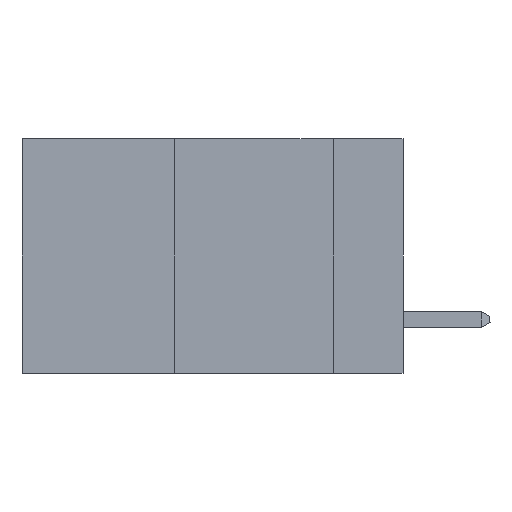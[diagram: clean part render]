
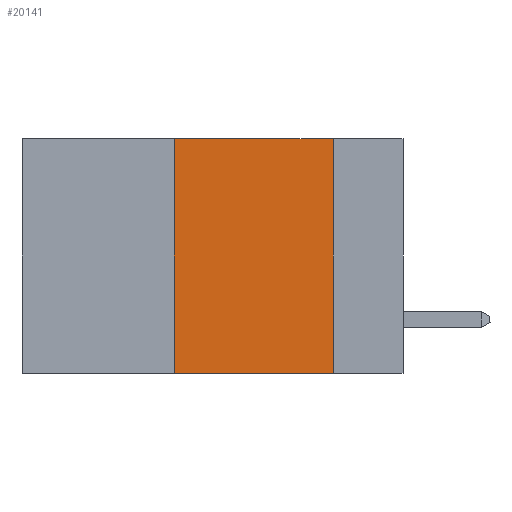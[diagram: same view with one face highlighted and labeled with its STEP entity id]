
A CAD part, left-side view. The second image highlights one B-rep face of the part: STEP entity #20141.
In plain terms, the highlighted planar face has unit normal (-1, 0, 0).
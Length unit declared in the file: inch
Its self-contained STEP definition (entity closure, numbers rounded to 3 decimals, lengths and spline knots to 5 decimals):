
#203 = VERTEX_POINT ( 'NONE', #24056 ) ;
#436 = DIRECTION ( 'NONE',  ( 0., 0., -1. ) ) ;
#682 = LINE ( 'NONE', #20265, #16203 ) ;
#1574 = ORIENTED_EDGE ( 'NONE', *, *, #17843, .F. ) ;
#2087 = CARTESIAN_POINT ( 'NONE',  ( 0., 0.6, 0. ) ) ;
#3830 = EDGE_CURVE ( 'NONE', #203, #29675, #9218, .T. ) ;
#4509 = CARTESIAN_POINT ( 'NONE',  ( 0., 0.6, -0.37 ) ) ;
#5100 = CARTESIAN_POINT ( 'NONE',  ( 0., 0.11, -0.37 ) ) ;
#5851 = CARTESIAN_POINT ( 'NONE',  ( 0., 0.36, 0. ) ) ;
#6160 = AXIS2_PLACEMENT_3D ( 'NONE', #2087, #24772, #436 ) ;
#6168 = ORIENTED_EDGE ( 'NONE', *, *, #24095, .F. ) ;
#7681 = CARTESIAN_POINT ( 'NONE',  ( 0., 0.6, 0. ) ) ;
#9218 = LINE ( 'NONE', #5851, #25414 ) ;
#9729 = DIRECTION ( 'NONE',  ( 0., -1., 0. ) ) ;
#9740 = VERTEX_POINT ( 'NONE', #19807 ) ;
#10594 = VECTOR ( 'NONE', #11298, 39.37008 ) ;
#11052 = CARTESIAN_POINT ( 'NONE',  ( 0., 0.36, 0. ) ) ;
#11298 = DIRECTION ( 'NONE',  ( 0., -1., 0. ) ) ;
#12783 = EDGE_LOOP ( 'NONE', ( #6168, #1574, #18027, #19750 ) ) ;
#13774 = LINE ( 'NONE', #7681, #25275 ) ;
#16203 = VECTOR ( 'NONE', #20165, 39.37008 ) ;
#17843 = EDGE_CURVE ( 'NONE', #29675, #9740, #13774, .T. ) ;
#18027 = ORIENTED_EDGE ( 'NONE', *, *, #3830, .F. ) ;
#19053 = VERTEX_POINT ( 'NONE', #5100 ) ;
#19750 = ORIENTED_EDGE ( 'NONE', *, *, #27421, .T. ) ;
#19807 = CARTESIAN_POINT ( 'NONE',  ( 0., 0.11, 0. ) ) ;
#20141 = ADVANCED_FACE ( 'NONE', ( #29139 ), #20319, .F. ) ;
#20165 = DIRECTION ( 'NONE',  ( 0., 0., -1. ) ) ;
#20265 = CARTESIAN_POINT ( 'NONE',  ( 0., 0.11, 0. ) ) ;
#20319 = PLANE ( 'NONE',  #6160 ) ;
#24056 = CARTESIAN_POINT ( 'NONE',  ( 0., 0.36, -0.37 ) ) ;
#24095 = EDGE_CURVE ( 'NONE', #9740, #19053, #682, .T. ) ;
#24499 = DIRECTION ( 'NONE',  ( 0., 0., 1. ) ) ;
#24772 = DIRECTION ( 'NONE',  ( 1., 0., 0. ) ) ;
#25011 = LINE ( 'NONE', #4509, #10594 ) ;
#25275 = VECTOR ( 'NONE', #9729, 39.37008 ) ;
#25414 = VECTOR ( 'NONE', #24499, 39.37008 ) ;
#27421 = EDGE_CURVE ( 'NONE', #203, #19053, #25011, .T. ) ;
#29139 = FACE_OUTER_BOUND ( 'NONE', #12783, .T. ) ;
#29675 = VERTEX_POINT ( 'NONE', #11052 ) ;
